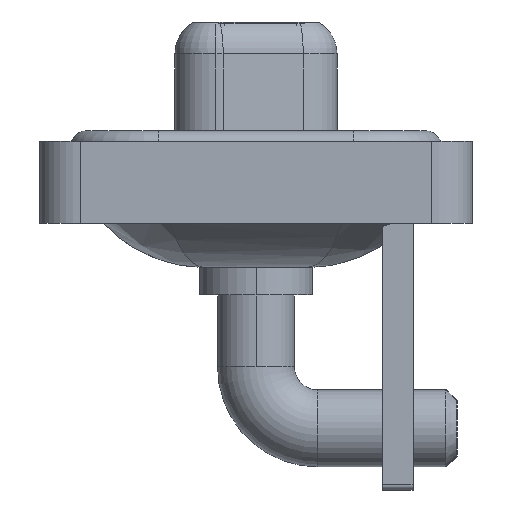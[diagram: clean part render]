
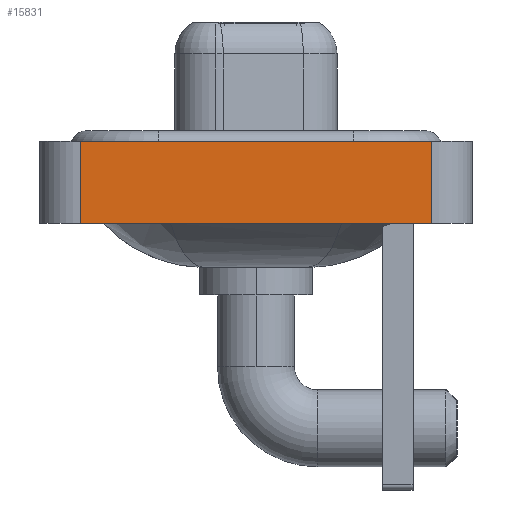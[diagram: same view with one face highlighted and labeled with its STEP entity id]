
A CAD part, left-side view. The second image highlights one B-rep face of the part: STEP entity #15831.
In plain terms, the highlighted planar face has unit normal (-1, 0, 0).
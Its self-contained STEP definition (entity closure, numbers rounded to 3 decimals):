
#60 = CARTESIAN_POINT ( 'NONE',  ( -7.25, 8.55, -3.6 ) ) ;
#449 = CARTESIAN_POINT ( 'NONE',  ( -7.25, -8.55, -3.6 ) ) ;
#1008 = EDGE_LOOP ( 'NONE', ( #10001, #13608, #10830, #8494 ) ) ;
#1929 = DIRECTION ( 'NONE',  ( -1., 0., 0. ) ) ;
#2574 = VERTEX_POINT ( 'NONE', #14928 ) ;
#2728 = CARTESIAN_POINT ( 'NONE',  ( -7.25, 8.55, -3.6 ) ) ;
#2782 = VERTEX_POINT ( 'NONE', #7459 ) ;
#2843 = CARTESIAN_POINT ( 'NONE',  ( -7.25, -8.55, -3.6 ) ) ;
#3868 = VECTOR ( 'NONE', #6680, 1000. ) ;
#4045 = VECTOR ( 'NONE', #17376, 1000. ) ;
#4910 = CARTESIAN_POINT ( 'NONE',  ( -7.25, -8.55, 0.4 ) ) ;
#5179 = CARTESIAN_POINT ( 'NONE',  ( -7.25, -8.55, -3.6 ) ) ;
#5298 = EDGE_CURVE ( 'NONE', #9991, #2574, #9451, .T. ) ;
#6680 = DIRECTION ( 'NONE',  ( 0., -1., 0. ) ) ;
#7459 = CARTESIAN_POINT ( 'NONE',  ( -7.25, -8.55, 0.4 ) ) ;
#7495 = LINE ( 'NONE', #4910, #14667 ) ;
#7575 = VECTOR ( 'NONE', #11396, 1000. ) ;
#7660 = CARTESIAN_POINT ( 'NONE',  ( -7.25, -8.55, -3.6 ) ) ;
#8494 = ORIENTED_EDGE ( 'NONE', *, *, #12840, .T. ) ;
#8737 = PLANE ( 'NONE',  #11320 ) ;
#9451 = LINE ( 'NONE', #2728, #4045 ) ;
#9991 = VERTEX_POINT ( 'NONE', #60 ) ;
#10001 = ORIENTED_EDGE ( 'NONE', *, *, #13516, .T. ) ;
#10830 = ORIENTED_EDGE ( 'NONE', *, *, #5298, .F. ) ;
#11320 = AXIS2_PLACEMENT_3D ( 'NONE', #7660, #1929, #13059 ) ;
#11396 = DIRECTION ( 'NONE',  ( 0., 0., 1. ) ) ;
#11419 = EDGE_CURVE ( 'NONE', #2574, #2782, #7495, .T. ) ;
#11540 = DIRECTION ( 'NONE',  ( 0., -1., 0. ) ) ;
#12734 = LINE ( 'NONE', #449, #7575 ) ;
#12840 = EDGE_CURVE ( 'NONE', #9991, #17083, #16204, .T. ) ;
#13059 = DIRECTION ( 'NONE',  ( 0., 0., 1. ) ) ;
#13147 = FACE_OUTER_BOUND ( 'NONE', #1008, .T. ) ;
#13516 = EDGE_CURVE ( 'NONE', #17083, #2782, #12734, .T. ) ;
#13608 = ORIENTED_EDGE ( 'NONE', *, *, #11419, .F. ) ;
#14667 = VECTOR ( 'NONE', #11540, 1000. ) ;
#14928 = CARTESIAN_POINT ( 'NONE',  ( -7.25, 8.55, 0.4 ) ) ;
#15831 = ADVANCED_FACE ( 'NONE', ( #13147 ), #8737, .T. ) ;
#16204 = LINE ( 'NONE', #5179, #3868 ) ;
#17083 = VERTEX_POINT ( 'NONE', #2843 ) ;
#17376 = DIRECTION ( 'NONE',  ( 0., 0., 1. ) ) ;
